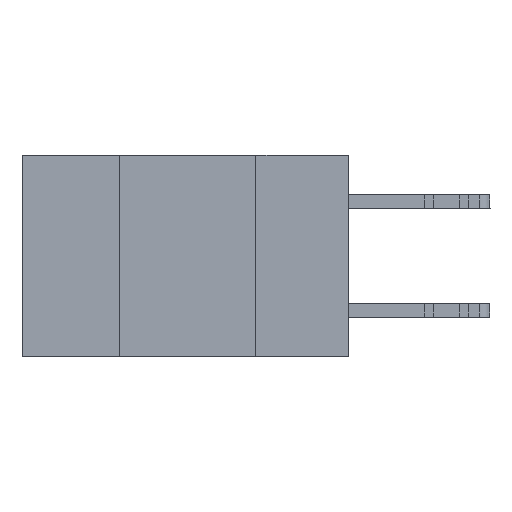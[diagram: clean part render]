
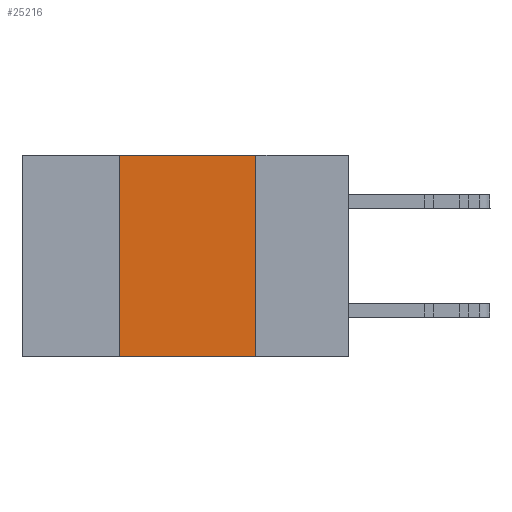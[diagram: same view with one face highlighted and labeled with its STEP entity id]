
A CAD part, left-side view. The second image highlights one B-rep face of the part: STEP entity #25216.
In plain terms, the highlighted planar face has unit normal (-1, 0, 0).
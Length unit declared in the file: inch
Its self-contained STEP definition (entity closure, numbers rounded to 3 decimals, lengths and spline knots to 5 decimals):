
#824 = LINE ( 'NONE', #1613, #20717 ) ;
#1326 = CARTESIAN_POINT ( 'NONE',  ( 0., 0.17, -0.37 ) ) ;
#1613 = CARTESIAN_POINT ( 'NONE',  ( 0., 0.6, 0. ) ) ;
#1654 = VECTOR ( 'NONE', #24874, 39.37008 ) ;
#2678 = CARTESIAN_POINT ( 'NONE',  ( 0., 0.17, 0. ) ) ;
#3024 = DIRECTION ( 'NONE',  ( 0., -1., 0. ) ) ;
#4902 = EDGE_CURVE ( 'NONE', #14313, #26696, #20616, .T. ) ;
#7317 = CARTESIAN_POINT ( 'NONE',  ( 0., 0.6, -0.37 ) ) ;
#7754 = PLANE ( 'NONE',  #18156 ) ;
#9519 = LINE ( 'NONE', #22295, #1654 ) ;
#10177 = VERTEX_POINT ( 'NONE', #20703 ) ;
#13256 = DIRECTION ( 'NONE',  ( 0., -1., 0. ) ) ;
#13885 = VERTEX_POINT ( 'NONE', #2678 ) ;
#14205 = DIRECTION ( 'NONE',  ( 0., 0., -1. ) ) ;
#14313 = VERTEX_POINT ( 'NONE', #22735 ) ;
#14769 = EDGE_CURVE ( 'NONE', #13885, #26696, #15565, .T. ) ;
#15366 = ORIENTED_EDGE ( 'NONE', *, *, #21118, .F. ) ;
#15565 = LINE ( 'NONE', #23193, #19844 ) ;
#16420 = ORIENTED_EDGE ( 'NONE', *, *, #14769, .F. ) ;
#18156 = AXIS2_PLACEMENT_3D ( 'NONE', #23740, #21148, #14205 ) ;
#19844 = VECTOR ( 'NONE', #20920, 39.37008 ) ;
#20616 = LINE ( 'NONE', #7317, #23089 ) ;
#20703 = CARTESIAN_POINT ( 'NONE',  ( 0., 0.42, 0. ) ) ;
#20717 = VECTOR ( 'NONE', #13256, 39.37008 ) ;
#20920 = DIRECTION ( 'NONE',  ( 0., 0., -1. ) ) ;
#21118 = EDGE_CURVE ( 'NONE', #14313, #10177, #9519, .T. ) ;
#21148 = DIRECTION ( 'NONE',  ( 1., 0., 0. ) ) ;
#22295 = CARTESIAN_POINT ( 'NONE',  ( 0., 0.42, 0. ) ) ;
#22495 = ORIENTED_EDGE ( 'NONE', *, *, #4902, .T. ) ;
#22735 = CARTESIAN_POINT ( 'NONE',  ( 0., 0.42, -0.37 ) ) ;
#23089 = VECTOR ( 'NONE', #3024, 39.37008 ) ;
#23193 = CARTESIAN_POINT ( 'NONE',  ( 0., 0.17, 0. ) ) ;
#23740 = CARTESIAN_POINT ( 'NONE',  ( 0., 0.6, 0. ) ) ;
#24667 = ORIENTED_EDGE ( 'NONE', *, *, #26015, .F. ) ;
#24874 = DIRECTION ( 'NONE',  ( 0., 0., 1. ) ) ;
#25216 = ADVANCED_FACE ( 'NONE', ( #26994 ), #7754, .F. ) ;
#26015 = EDGE_CURVE ( 'NONE', #10177, #13885, #824, .T. ) ;
#26082 = EDGE_LOOP ( 'NONE', ( #16420, #24667, #15366, #22495 ) ) ;
#26696 = VERTEX_POINT ( 'NONE', #1326 ) ;
#26994 = FACE_OUTER_BOUND ( 'NONE', #26082, .T. ) ;
